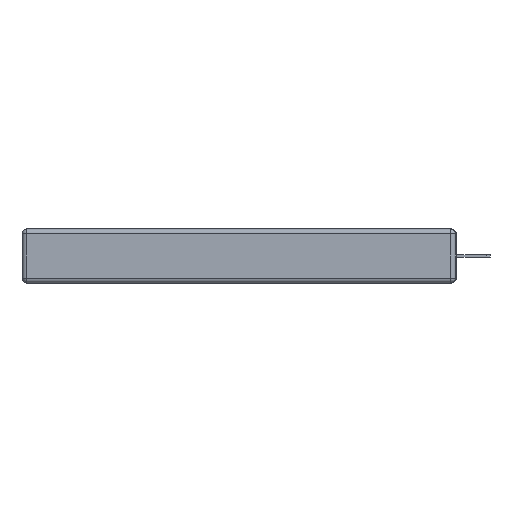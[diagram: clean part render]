
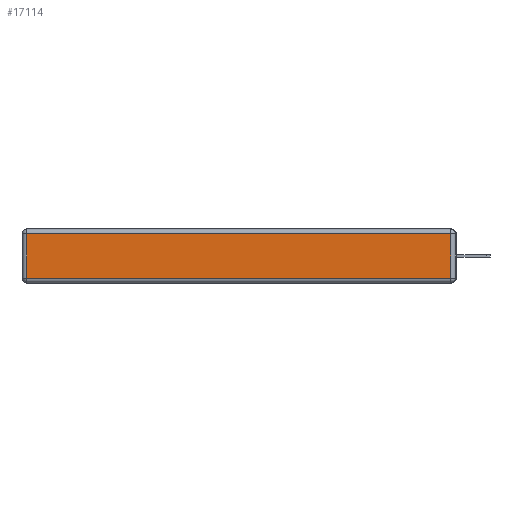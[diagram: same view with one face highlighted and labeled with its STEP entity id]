
A CAD part, left-side view. The second image highlights one B-rep face of the part: STEP entity #17114.
In plain terms, the highlighted planar face has unit normal (-1, 0, 0).
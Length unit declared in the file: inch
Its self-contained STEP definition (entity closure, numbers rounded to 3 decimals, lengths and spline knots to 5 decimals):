
#112 = FACE_OUTER_BOUND ( 'NONE', #16311, .T. ) ;
#253 = EDGE_CURVE ( 'NONE', #5060, #23551, #6781, .T. ) ;
#1224 = VECTOR ( 'NONE', #14490, 39.37008 ) ;
#4732 = VECTOR ( 'NONE', #20927, 39.37008 ) ;
#5024 = DIRECTION ( 'NONE',  ( 0., 0., 1. ) ) ;
#5060 = VERTEX_POINT ( 'NONE', #16630 ) ;
#6450 = EDGE_CURVE ( 'NONE', #24009, #9476, #8526, .T. ) ;
#6781 = LINE ( 'NONE', #16480, #4732 ) ;
#6903 = VECTOR ( 'NONE', #9479, 39.37008 ) ;
#7040 = CARTESIAN_POINT ( 'NONE',  ( 0., 0.03, -0.03 ) ) ;
#7819 = VECTOR ( 'NONE', #8035, 39.37008 ) ;
#8035 = DIRECTION ( 'NONE',  ( 0., 1., 0. ) ) ;
#8197 = EDGE_CURVE ( 'NONE', #9476, #5060, #23045, .T. ) ;
#8526 = LINE ( 'NONE', #21012, #7819 ) ;
#9323 = DIRECTION ( 'NONE',  ( -1., 0., 0. ) ) ;
#9476 = VERTEX_POINT ( 'NONE', #16809 ) ;
#9479 = DIRECTION ( 'NONE',  ( 0., 0., 1. ) ) ;
#9510 = CARTESIAN_POINT ( 'NONE',  ( 0., 0., -0.343 ) ) ;
#10504 = ORIENTED_EDGE ( 'NONE', *, *, #253, .T. ) ;
#10876 = PLANE ( 'NONE',  #20622 ) ;
#11479 = ORIENTED_EDGE ( 'NONE', *, *, #6450, .T. ) ;
#12011 = LINE ( 'NONE', #22582, #6903 ) ;
#12379 = CARTESIAN_POINT ( 'NONE',  ( 0., 2.72, -0.343 ) ) ;
#14490 = DIRECTION ( 'NONE',  ( 0., 0., -1. ) ) ;
#16311 = EDGE_LOOP ( 'NONE', ( #10504, #23215, #11479, #18292 ) ) ;
#16480 = CARTESIAN_POINT ( 'NONE',  ( 0., 0., -0.313 ) ) ;
#16630 = CARTESIAN_POINT ( 'NONE',  ( 0., 2.72, -0.313 ) ) ;
#16809 = CARTESIAN_POINT ( 'NONE',  ( 0., 2.72, -0.03 ) ) ;
#16846 = EDGE_CURVE ( 'NONE', #23551, #24009, #12011, .T. ) ;
#17114 = ADVANCED_FACE ( 'NONE', ( #112 ), #10876, .T. ) ;
#18292 = ORIENTED_EDGE ( 'NONE', *, *, #8197, .T. ) ;
#20622 = AXIS2_PLACEMENT_3D ( 'NONE', #9510, #9323, #5024 ) ;
#20927 = DIRECTION ( 'NONE',  ( 0., -1., 0. ) ) ;
#21012 = CARTESIAN_POINT ( 'NONE',  ( 0., 2.75, -0.03 ) ) ;
#22582 = CARTESIAN_POINT ( 'NONE',  ( 0., 0.03, -0.343 ) ) ;
#23045 = LINE ( 'NONE', #12379, #1224 ) ;
#23215 = ORIENTED_EDGE ( 'NONE', *, *, #16846, .T. ) ;
#23551 = VERTEX_POINT ( 'NONE', #24873 ) ;
#24009 = VERTEX_POINT ( 'NONE', #7040 ) ;
#24873 = CARTESIAN_POINT ( 'NONE',  ( 0., 0.03, -0.313 ) ) ;
